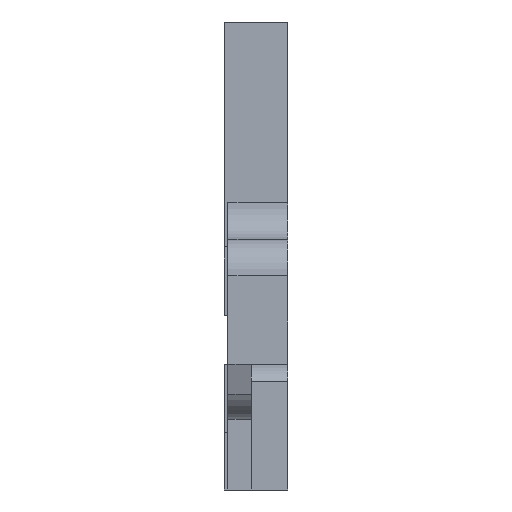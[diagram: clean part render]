
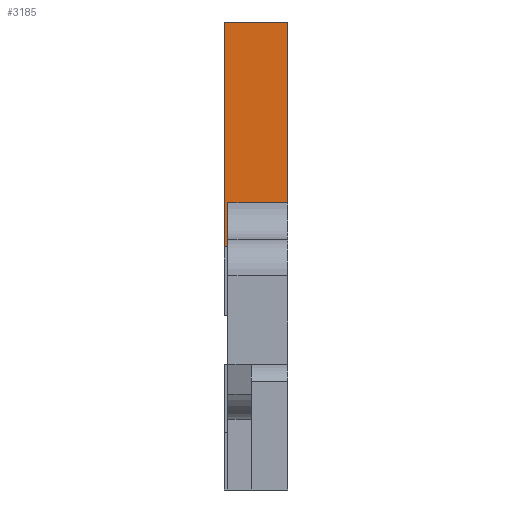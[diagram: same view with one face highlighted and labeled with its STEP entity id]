
A CAD part, left-side view. The second image highlights one B-rep face of the part: STEP entity #3185.
In plain terms, the highlighted planar face has unit normal (-1, 0, 0).
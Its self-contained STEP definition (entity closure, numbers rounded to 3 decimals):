
#218 = DIRECTION ( 'NONE',  ( 0., -1., 0. ) ) ;
#279 = VERTEX_POINT ( 'NONE', #3446 ) ;
#663 = CARTESIAN_POINT ( 'NONE',  ( -1.5, -0.533, -24.88 ) ) ;
#732 = VERTEX_POINT ( 'NONE', #5537 ) ;
#966 = VERTEX_POINT ( 'NONE', #9063 ) ;
#1025 = VECTOR ( 'NONE', #218, 1000. ) ;
#1264 = CARTESIAN_POINT ( 'NONE',  ( -1.5, 29.762, 0. ) ) ;
#1424 = EDGE_CURVE ( 'NONE', #279, #966, #10199, .T. ) ;
#1453 = DIRECTION ( 'NONE',  ( 0., -1., 0. ) ) ;
#1502 = DIRECTION ( 'NONE',  ( 0., 0., 1. ) ) ;
#1901 = EDGE_CURVE ( 'NONE', #9679, #3964, #11098, .T. ) ;
#1940 = CARTESIAN_POINT ( 'NONE',  ( -1.5, 29.762, 0. ) ) ;
#2065 = DIRECTION ( 'NONE',  ( -1., 0., 0. ) ) ;
#2488 = ORIENTED_EDGE ( 'NONE', *, *, #4102, .T. ) ;
#2589 = LINE ( 'NONE', #10396, #3664 ) ;
#3185 = ADVANCED_FACE ( 'NONE', ( #8962 ), #4863, .T. ) ;
#3330 = LINE ( 'NONE', #9874, #1025 ) ;
#3446 = CARTESIAN_POINT ( 'NONE',  ( -1.5, -0.533, -30.931 ) ) ;
#3664 = VECTOR ( 'NONE', #11344, 1000. ) ;
#3775 = VECTOR ( 'NONE', #1502, 1000. ) ;
#3856 = CARTESIAN_POINT ( 'NONE',  ( -1.5, -8.783, -24.88 ) ) ;
#3887 = ORIENTED_EDGE ( 'NONE', *, *, #5832, .F. ) ;
#3964 = VERTEX_POINT ( 'NONE', #4357 ) ;
#4102 = EDGE_CURVE ( 'NONE', #732, #279, #11388, .T. ) ;
#4357 = CARTESIAN_POINT ( 'NONE',  ( -1.5, -8.783, 0. ) ) ;
#4863 = PLANE ( 'NONE',  #11014 ) ;
#5537 = CARTESIAN_POINT ( 'NONE',  ( -1.5, -0.029, -30.931 ) ) ;
#5832 = EDGE_CURVE ( 'NONE', #3964, #10236, #2589, .T. ) ;
#5973 = EDGE_CURVE ( 'NONE', #732, #9679, #6923, .T. ) ;
#6066 = ORIENTED_EDGE ( 'NONE', *, *, #1901, .F. ) ;
#6410 = EDGE_CURVE ( 'NONE', #966, #10236, #3330, .T. ) ;
#6778 = CARTESIAN_POINT ( 'NONE',  ( -1.5, 30.937, -30.931 ) ) ;
#6923 = LINE ( 'NONE', #9829, #9121 ) ;
#7811 = DIRECTION ( 'NONE',  ( 0., 0., 1. ) ) ;
#7834 = ORIENTED_EDGE ( 'NONE', *, *, #6410, .T. ) ;
#8037 = EDGE_LOOP ( 'NONE', ( #10422, #7834, #3887, #6066, #9168, #2488 ) ) ;
#8962 = FACE_OUTER_BOUND ( 'NONE', #8037, .T. ) ;
#9063 = CARTESIAN_POINT ( 'NONE',  ( -1.5, -0.533, -24.88 ) ) ;
#9121 = VECTOR ( 'NONE', #7811, 1000. ) ;
#9168 = ORIENTED_EDGE ( 'NONE', *, *, #5973, .F. ) ;
#9679 = VERTEX_POINT ( 'NONE', #12515 ) ;
#9829 = CARTESIAN_POINT ( 'NONE',  ( -1.5, -0.029, -24.88 ) ) ;
#9874 = CARTESIAN_POINT ( 'NONE',  ( -1.5, -8.783, -24.88 ) ) ;
#10199 = LINE ( 'NONE', #663, #3775 ) ;
#10236 = VERTEX_POINT ( 'NONE', #3856 ) ;
#10396 = CARTESIAN_POINT ( 'NONE',  ( -1.5, -8.783, 0. ) ) ;
#10422 = ORIENTED_EDGE ( 'NONE', *, *, #1424, .T. ) ;
#11014 = AXIS2_PLACEMENT_3D ( 'NONE', #1940, #2065, #11831 ) ;
#11098 = LINE ( 'NONE', #1264, #11350 ) ;
#11344 = DIRECTION ( 'NONE',  ( 0., 0., -1. ) ) ;
#11350 = VECTOR ( 'NONE', #1453, 1000. ) ;
#11388 = LINE ( 'NONE', #6778, #11560 ) ;
#11560 = VECTOR ( 'NONE', #12337, 1000. ) ;
#11831 = DIRECTION ( 'NONE',  ( 0., 0., 1. ) ) ;
#12337 = DIRECTION ( 'NONE',  ( 0., -1., 0. ) ) ;
#12515 = CARTESIAN_POINT ( 'NONE',  ( -1.5, -0.029, 0. ) ) ;
